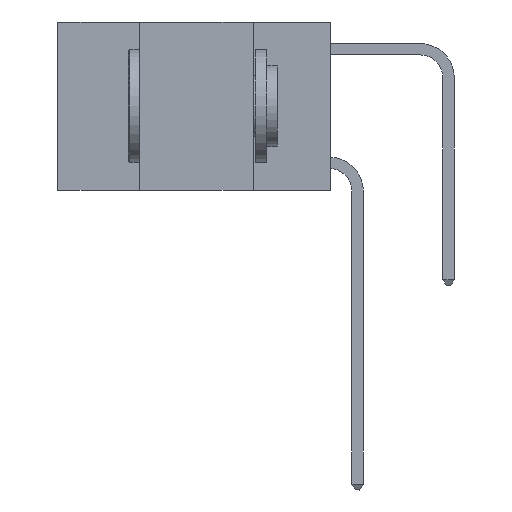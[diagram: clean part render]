
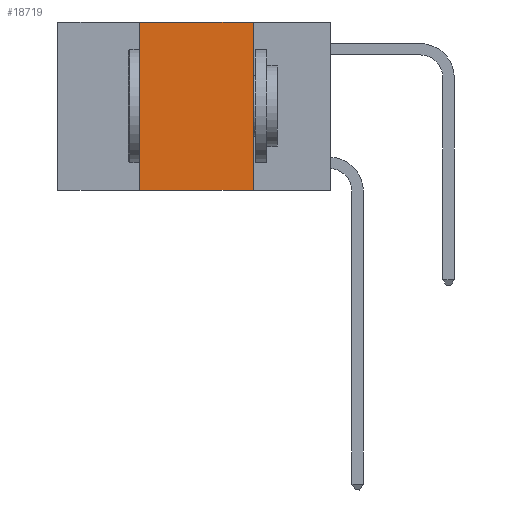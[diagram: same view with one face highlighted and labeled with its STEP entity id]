
A CAD part, left-side view. The second image highlights one B-rep face of the part: STEP entity #18719.
In plain terms, the highlighted planar face has unit normal (-1, 0, 0).
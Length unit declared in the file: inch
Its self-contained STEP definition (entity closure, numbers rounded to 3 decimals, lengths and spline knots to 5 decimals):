
#850 = DIRECTION ( 'NONE',  ( 0., -1., 0. ) ) ;
#1725 = PLANE ( 'NONE',  #9785 ) ;
#2850 = CARTESIAN_POINT ( 'NONE',  ( 0., 0.17, 0. ) ) ;
#3157 = EDGE_CURVE ( 'NONE', #7591, #19778, #20981, .T. ) ;
#3280 = VERTEX_POINT ( 'NONE', #19273 ) ;
#3495 = DIRECTION ( 'NONE',  ( 1., 0., 0. ) ) ;
#3523 = DIRECTION ( 'NONE',  ( 0., 0., 1. ) ) ;
#4616 = FACE_OUTER_BOUND ( 'NONE', #11839, .T. ) ;
#4771 = ORIENTED_EDGE ( 'NONE', *, *, #20312, .T. ) ;
#4931 = DIRECTION ( 'NONE',  ( 0., -1., 0. ) ) ;
#5481 = EDGE_CURVE ( 'NONE', #3280, #13199, #17251, .T. ) ;
#6802 = VECTOR ( 'NONE', #3523, 39.37008 ) ;
#7591 = VERTEX_POINT ( 'NONE', #10467 ) ;
#7797 = ORIENTED_EDGE ( 'NONE', *, *, #5481, .F. ) ;
#8936 = VECTOR ( 'NONE', #4931, 39.37008 ) ;
#9785 = AXIS2_PLACEMENT_3D ( 'NONE', #12181, #3495, #15616 ) ;
#10146 = EDGE_CURVE ( 'NONE', #19778, #3280, #10393, .T. ) ;
#10393 = LINE ( 'NONE', #13047, #18932 ) ;
#10467 = CARTESIAN_POINT ( 'NONE',  ( 0., 0.42, -0.37 ) ) ;
#10474 = CARTESIAN_POINT ( 'NONE',  ( 0., 0.42, 0. ) ) ;
#11839 = EDGE_LOOP ( 'NONE', ( #7797, #12947, #21926, #4771 ) ) ;
#12181 = CARTESIAN_POINT ( 'NONE',  ( 0., 0.6, 0. ) ) ;
#12305 = CARTESIAN_POINT ( 'NONE',  ( 0., 0.17, -0.37 ) ) ;
#12433 = LINE ( 'NONE', #20402, #8936 ) ;
#12947 = ORIENTED_EDGE ( 'NONE', *, *, #10146, .F. ) ;
#13047 = CARTESIAN_POINT ( 'NONE',  ( 0., 0.6, 0. ) ) ;
#13199 = VERTEX_POINT ( 'NONE', #12305 ) ;
#15616 = DIRECTION ( 'NONE',  ( 0., 0., -1. ) ) ;
#15639 = VECTOR ( 'NONE', #21674, 39.37008 ) ;
#17251 = LINE ( 'NONE', #2850, #15639 ) ;
#18719 = ADVANCED_FACE ( 'NONE', ( #4616 ), #1725, .F. ) ;
#18932 = VECTOR ( 'NONE', #850, 39.37008 ) ;
#19273 = CARTESIAN_POINT ( 'NONE',  ( 0., 0.17, 0. ) ) ;
#19778 = VERTEX_POINT ( 'NONE', #20854 ) ;
#20312 = EDGE_CURVE ( 'NONE', #7591, #13199, #12433, .T. ) ;
#20402 = CARTESIAN_POINT ( 'NONE',  ( 0., 0.6, -0.37 ) ) ;
#20854 = CARTESIAN_POINT ( 'NONE',  ( 0., 0.42, 0. ) ) ;
#20981 = LINE ( 'NONE', #10474, #6802 ) ;
#21674 = DIRECTION ( 'NONE',  ( 0., 0., -1. ) ) ;
#21926 = ORIENTED_EDGE ( 'NONE', *, *, #3157, .F. ) ;
